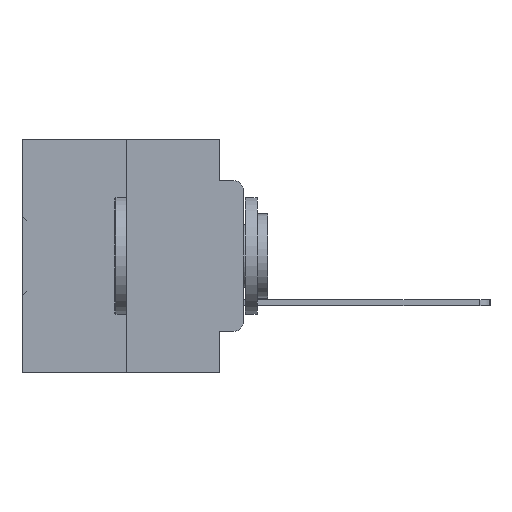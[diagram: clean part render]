
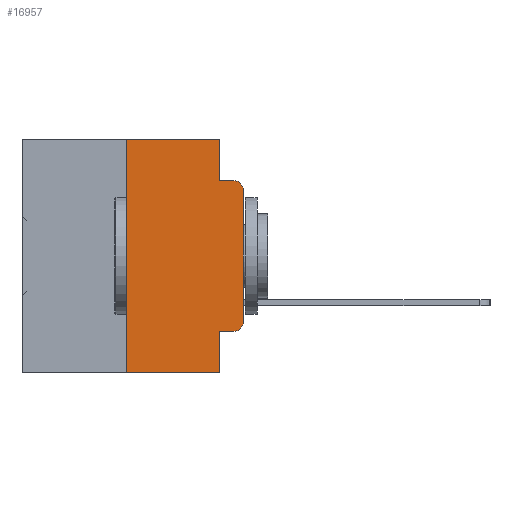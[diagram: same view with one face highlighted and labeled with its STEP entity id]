
A CAD part, left-side view. The second image highlights one B-rep face of the part: STEP entity #16957.
In plain terms, the highlighted planar face has unit normal (-1, 0, 0).
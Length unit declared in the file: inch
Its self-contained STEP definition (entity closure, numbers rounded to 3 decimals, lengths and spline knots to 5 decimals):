
#181 = EDGE_CURVE ( 'NONE', #13256, #29890, #5066, .T. ) ;
#654 = DIRECTION ( 'NONE',  ( -1., 0., 0. ) ) ;
#828 = VECTOR ( 'NONE', #11163, 39.37008 ) ;
#2251 = ORIENTED_EDGE ( 'NONE', *, *, #23189, .F. ) ;
#2340 = VERTEX_POINT ( 'NONE', #16519 ) ;
#2629 = VERTEX_POINT ( 'NONE', #12025 ) ;
#3172 = DIRECTION ( 'NONE',  ( 1., 0., 0. ) ) ;
#3840 = CARTESIAN_POINT ( 'NONE',  ( 0., 0.051, -0.5 ) ) ;
#3964 = CARTESIAN_POINT ( 'NONE',  ( 0., 0.02, -0.1085 ) ) ;
#5020 = ORIENTED_EDGE ( 'NONE', *, *, #21105, .T. ) ;
#5066 = CIRCLE ( 'NONE', #31702, 0.02 ) ;
#5587 = LINE ( 'NONE', #22498, #34711 ) ;
#5907 = CARTESIAN_POINT ( 'NONE',  ( 0., 0., 0. ) ) ;
#5956 = ORIENTED_EDGE ( 'NONE', *, *, #181, .T. ) ;
#6840 = ORIENTED_EDGE ( 'NONE', *, *, #11846, .F. ) ;
#6908 = DIRECTION ( 'NONE',  ( 0., 0., -1. ) ) ;
#7109 = DIRECTION ( 'NONE',  ( 0., 0., -1. ) ) ;
#7170 = CARTESIAN_POINT ( 'NONE',  ( 0., 0.25, 0. ) ) ;
#7480 = FACE_OUTER_BOUND ( 'NONE', #24175, .T. ) ;
#9205 = CARTESIAN_POINT ( 'NONE',  ( 0., 0.051, -0.4115 ) ) ;
#9266 = AXIS2_PLACEMENT_3D ( 'NONE', #14572, #3172, #23035 ) ;
#9411 = CIRCLE ( 'NONE', #17967, 0.02 ) ;
#9931 = EDGE_CURVE ( 'NONE', #33126, #13256, #26200, .T. ) ;
#10373 = CARTESIAN_POINT ( 'NONE',  ( 0., 0.051, -0.0885 ) ) ;
#11163 = DIRECTION ( 'NONE',  ( 0., -1., 0. ) ) ;
#11196 = VECTOR ( 'NONE', #27990, 39.37008 ) ;
#11252 = DIRECTION ( 'NONE',  ( 0., 0., -1. ) ) ;
#11632 = DIRECTION ( 'NONE',  ( 0., 0., -1. ) ) ;
#11846 = EDGE_CURVE ( 'NONE', #33126, #34465, #5587, .T. ) ;
#12025 = CARTESIAN_POINT ( 'NONE',  ( 0., 0.02, -0.0885 ) ) ;
#12541 = CARTESIAN_POINT ( 'NONE',  ( 0., 0.02, -0.3915 ) ) ;
#12770 = CARTESIAN_POINT ( 'NONE',  ( 0., 0.25, 0. ) ) ;
#13042 = ORIENTED_EDGE ( 'NONE', *, *, #32588, .T. ) ;
#13120 = LINE ( 'NONE', #36092, #33778 ) ;
#13256 = VERTEX_POINT ( 'NONE', #22840 ) ;
#14398 = CARTESIAN_POINT ( 'NONE',  ( 0., 0.051, 0. ) ) ;
#14572 = CARTESIAN_POINT ( 'NONE',  ( 0., 0.473, 0. ) ) ;
#14698 = VERTEX_POINT ( 'NONE', #12770 ) ;
#16265 = VECTOR ( 'NONE', #11632, 39.37008 ) ;
#16519 = CARTESIAN_POINT ( 'NONE',  ( 0., 0.25, -0.5 ) ) ;
#16957 = ADVANCED_FACE ( 'NONE', ( #7480 ), #17409, .F. ) ;
#17409 = PLANE ( 'NONE',  #9266 ) ;
#17967 = AXIS2_PLACEMENT_3D ( 'NONE', #3964, #23807, #6908 ) ;
#18019 = LINE ( 'NONE', #14398, #16265 ) ;
#19341 = VECTOR ( 'NONE', #26995, 39.37008 ) ;
#19420 = EDGE_CURVE ( 'NONE', #2340, #14698, #35166, .T. ) ;
#19436 = CARTESIAN_POINT ( 'NONE',  ( 0., 0., -0.3915 ) ) ;
#20583 = LINE ( 'NONE', #10373, #27132 ) ;
#21105 = EDGE_CURVE ( 'NONE', #2340, #34465, #23610, .T. ) ;
#21744 = DIRECTION ( 'NONE',  ( 0., -1., 0. ) ) ;
#22273 = CARTESIAN_POINT ( 'NONE',  ( 0., 0.051, -0.0885 ) ) ;
#22293 = ORIENTED_EDGE ( 'NONE', *, *, #26933, .F. ) ;
#22498 = CARTESIAN_POINT ( 'NONE',  ( 0., 0.051, 0. ) ) ;
#22766 = CARTESIAN_POINT ( 'NONE',  ( 0., 0., -0.1085 ) ) ;
#22840 = CARTESIAN_POINT ( 'NONE',  ( 0., 0.02, -0.4115 ) ) ;
#23035 = DIRECTION ( 'NONE',  ( 0., 0., -1. ) ) ;
#23044 = VERTEX_POINT ( 'NONE', #22273 ) ;
#23189 = EDGE_CURVE ( 'NONE', #25010, #23044, #18019, .T. ) ;
#23610 = LINE ( 'NONE', #28019, #828 ) ;
#23807 = DIRECTION ( 'NONE',  ( -1., 0., 0. ) ) ;
#24175 = EDGE_LOOP ( 'NONE', ( #34584, #13042, #22293, #2251, #24942, #34151, #5020, #6840, #33309, #5956 ) ) ;
#24594 = VERTEX_POINT ( 'NONE', #22766 ) ;
#24709 = CARTESIAN_POINT ( 'NONE',  ( 0., 0.051, 0. ) ) ;
#24942 = ORIENTED_EDGE ( 'NONE', *, *, #36619, .F. ) ;
#25010 = VERTEX_POINT ( 'NONE', #24709 ) ;
#25209 = CARTESIAN_POINT ( 'NONE',  ( 0., 0.051, -0.4115 ) ) ;
#25805 = VECTOR ( 'NONE', #34142, 39.37008 ) ;
#26200 = LINE ( 'NONE', #25209, #11196 ) ;
#26933 = EDGE_CURVE ( 'NONE', #23044, #2629, #20583, .T. ) ;
#26995 = DIRECTION ( 'NONE',  ( 0., 0., 1. ) ) ;
#27132 = VECTOR ( 'NONE', #21744, 39.37008 ) ;
#27713 = DIRECTION ( 'NONE',  ( 0., -1., 0. ) ) ;
#27990 = DIRECTION ( 'NONE',  ( 0., -1., 0. ) ) ;
#28019 = CARTESIAN_POINT ( 'NONE',  ( 0., 0.473, -0.5 ) ) ;
#29890 = VERTEX_POINT ( 'NONE', #19436 ) ;
#31702 = AXIS2_PLACEMENT_3D ( 'NONE', #12541, #654, #7109 ) ;
#31864 = EDGE_CURVE ( 'NONE', #29890, #24594, #33266, .T. ) ;
#32588 = EDGE_CURVE ( 'NONE', #24594, #2629, #9411, .T. ) ;
#33126 = VERTEX_POINT ( 'NONE', #9205 ) ;
#33266 = LINE ( 'NONE', #5907, #25805 ) ;
#33309 = ORIENTED_EDGE ( 'NONE', *, *, #9931, .T. ) ;
#33778 = VECTOR ( 'NONE', #27713, 39.37008 ) ;
#34142 = DIRECTION ( 'NONE',  ( 0., 0., 1. ) ) ;
#34151 = ORIENTED_EDGE ( 'NONE', *, *, #19420, .F. ) ;
#34465 = VERTEX_POINT ( 'NONE', #3840 ) ;
#34584 = ORIENTED_EDGE ( 'NONE', *, *, #31864, .T. ) ;
#34711 = VECTOR ( 'NONE', #11252, 39.37008 ) ;
#35166 = LINE ( 'NONE', #7170, #19341 ) ;
#36092 = CARTESIAN_POINT ( 'NONE',  ( 0., 0.473, 0. ) ) ;
#36619 = EDGE_CURVE ( 'NONE', #14698, #25010, #13120, .T. ) ;
